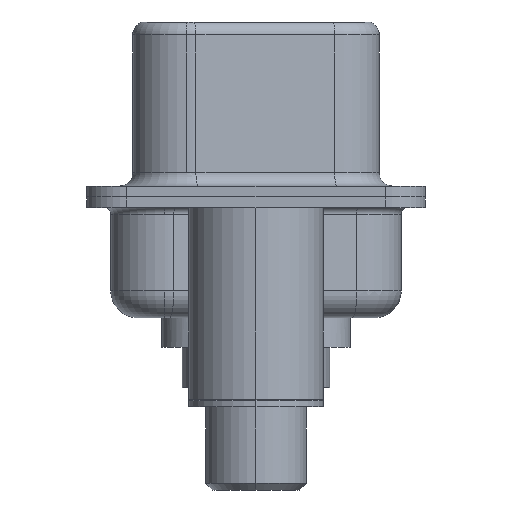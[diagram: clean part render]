
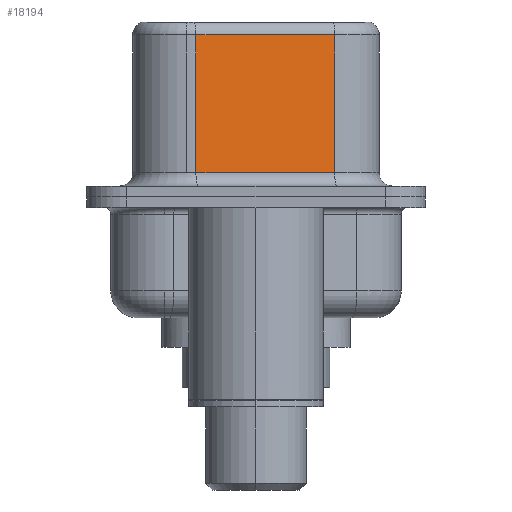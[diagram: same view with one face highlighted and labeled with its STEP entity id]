
A CAD part, left-side view. The second image highlights one B-rep face of the part: STEP entity #18194.
In plain terms, the highlighted planar face has unit normal (-0.985, -0.174, 0).
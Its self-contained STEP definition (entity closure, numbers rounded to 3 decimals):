
#97 = VECTOR ( 'NONE', #2236, 1000. ) ;
#1162 = EDGE_LOOP ( 'NONE', ( #17957, #3408, #8150, #17361 ) ) ;
#1273 = CARTESIAN_POINT ( 'NONE',  ( 4.58, -2.927, 6.52 ) ) ;
#1592 = DIRECTION ( 'NONE',  ( 0., 0., -1. ) ) ;
#1620 = LINE ( 'NONE', #17603, #5002 ) ;
#2193 = VERTEX_POINT ( 'NONE', #12628 ) ;
#2214 = EDGE_CURVE ( 'NONE', #16782, #6378, #6073, .T. ) ;
#2236 = DIRECTION ( 'NONE',  ( 0.174, -0.985, 0. ) ) ;
#2716 = DIRECTION ( 'NONE',  ( -0.174, 0.985, 0. ) ) ;
#3408 = ORIENTED_EDGE ( 'NONE', *, *, #2214, .T. ) ;
#3487 = CARTESIAN_POINT ( 'NONE',  ( 3.67, 2.233, 6.52 ) ) ;
#3492 = EDGE_CURVE ( 'NONE', #6378, #2193, #5590, .T. ) ;
#4131 = PLANE ( 'NONE',  #12115 ) ;
#5002 = VECTOR ( 'NONE', #7601, 1000. ) ;
#5590 = LINE ( 'NONE', #3487, #15632 ) ;
#5624 = VECTOR ( 'NONE', #17826, 1000. ) ;
#6073 = LINE ( 'NONE', #8227, #5624 ) ;
#6378 = VERTEX_POINT ( 'NONE', #11844 ) ;
#6590 = FACE_OUTER_BOUND ( 'NONE', #1162, .T. ) ;
#7601 = DIRECTION ( 'NONE',  ( 0., 0., -1. ) ) ;
#8049 = VERTEX_POINT ( 'NONE', #15431 ) ;
#8150 = ORIENTED_EDGE ( 'NONE', *, *, #3492, .T. ) ;
#8227 = CARTESIAN_POINT ( 'NONE',  ( 4.58, -2.927, 6.02 ) ) ;
#8637 = LINE ( 'NONE', #10912, #97 ) ;
#10912 = CARTESIAN_POINT ( 'NONE',  ( 4.58, -2.927, 0.9 ) ) ;
#11308 = DIRECTION ( 'NONE',  ( 0.985, 0.174, 0. ) ) ;
#11788 = CARTESIAN_POINT ( 'NONE',  ( 4.58, -2.927, 6.02 ) ) ;
#11844 = CARTESIAN_POINT ( 'NONE',  ( 3.67, 2.233, 6.02 ) ) ;
#11930 = EDGE_CURVE ( 'NONE', #16782, #8049, #1620, .T. ) ;
#12115 = AXIS2_PLACEMENT_3D ( 'NONE', #1273, #11308, #2716 ) ;
#12628 = CARTESIAN_POINT ( 'NONE',  ( 3.67, 2.233, 0.9 ) ) ;
#12796 = EDGE_CURVE ( 'NONE', #2193, #8049, #8637, .T. ) ;
#15431 = CARTESIAN_POINT ( 'NONE',  ( 4.58, -2.927, 0.9 ) ) ;
#15632 = VECTOR ( 'NONE', #1592, 1000. ) ;
#16782 = VERTEX_POINT ( 'NONE', #11788 ) ;
#17361 = ORIENTED_EDGE ( 'NONE', *, *, #12796, .T. ) ;
#17603 = CARTESIAN_POINT ( 'NONE',  ( 4.58, -2.927, 6.52 ) ) ;
#17826 = DIRECTION ( 'NONE',  ( -0.174, 0.985, 0. ) ) ;
#17957 = ORIENTED_EDGE ( 'NONE', *, *, #11930, .F. ) ;
#18194 = ADVANCED_FACE ( 'NONE', ( #6590 ), #4131, .F. ) ;
